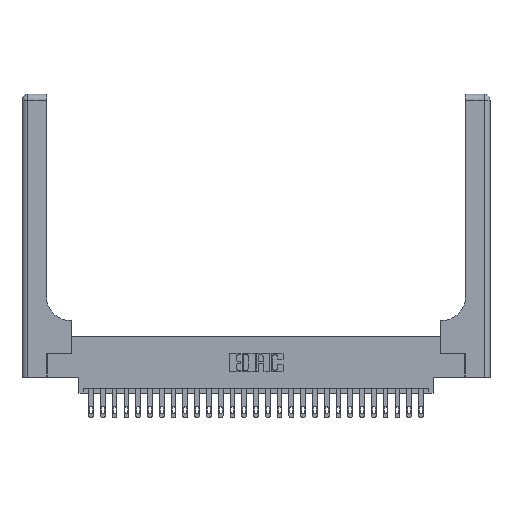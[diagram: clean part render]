
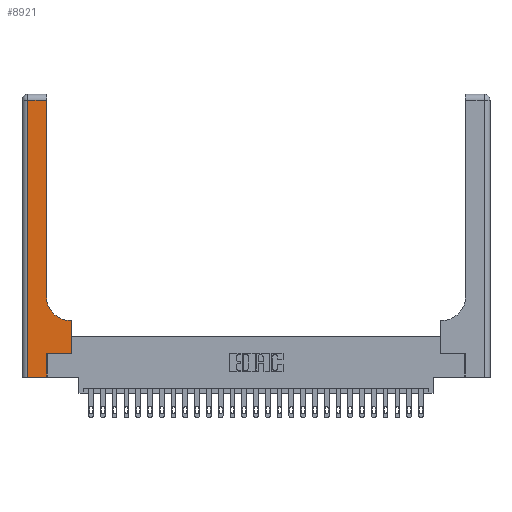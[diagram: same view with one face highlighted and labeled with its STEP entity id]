
A CAD part, top view. The second image highlights one B-rep face of the part: STEP entity #8921.
In plain terms, the highlighted planar face has unit normal (0, 0, 1).
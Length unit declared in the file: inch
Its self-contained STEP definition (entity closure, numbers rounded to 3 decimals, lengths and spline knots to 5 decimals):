
#951 = VECTOR ( 'NONE', #7399, 39.37008 ) ;
#977 = VERTEX_POINT ( 'NONE', #7825 ) ;
#1248 = EDGE_CURVE ( 'NONE', #22146, #21912, #2877, .T. ) ;
#1373 = VERTEX_POINT ( 'NONE', #18196 ) ;
#1767 = DIRECTION ( 'NONE',  ( -1., 0., 0. ) ) ;
#2043 = LINE ( 'NONE', #6017, #7101 ) ;
#2155 = EDGE_CURVE ( 'NONE', #2946, #977, #9315, .T. ) ;
#2622 = VERTEX_POINT ( 'NONE', #16186 ) ;
#2779 = AXIS2_PLACEMENT_3D ( 'NONE', #13784, #5751, #1767 ) ;
#2877 = LINE ( 'NONE', #7270, #951 ) ;
#2890 = VECTOR ( 'NONE', #3100, 39.37008 ) ;
#2946 = VERTEX_POINT ( 'NONE', #5224 ) ;
#3078 = CARTESIAN_POINT ( 'NONE',  ( 0.265, 0., 0.37 ) ) ;
#3100 = DIRECTION ( 'NONE',  ( 0., 1., 0. ) ) ;
#3441 = DIRECTION ( 'NONE',  ( 0., 1., 0. ) ) ;
#3541 = EDGE_CURVE ( 'NONE', #21912, #2622, #9478, .T. ) ;
#4646 = EDGE_CURVE ( 'NONE', #1373, #24744, #10700, .T. ) ;
#4874 = VECTOR ( 'NONE', #7732, 39.37008 ) ;
#5224 = CARTESIAN_POINT ( 'NONE',  ( 0.265, 0.25, 0.37 ) ) ;
#5430 = CARTESIAN_POINT ( 'NONE',  ( 0.26, 3., 0.37 ) ) ;
#5453 = CARTESIAN_POINT ( 'NONE',  ( 0.06, 3., 0.37 ) ) ;
#5552 = CARTESIAN_POINT ( 'NONE',  ( 0.265, 0.25, 0.37 ) ) ;
#5617 = PLANE ( 'NONE',  #2779 ) ;
#5751 = DIRECTION ( 'NONE',  ( 0., 0., -1. ) ) ;
#5753 = DIRECTION ( 'NONE',  ( -1., 0., 0. ) ) ;
#5936 = VECTOR ( 'NONE', #3441, 39.37008 ) ;
#6017 = CARTESIAN_POINT ( 'NONE',  ( 0., 0., 0.37 ) ) ;
#6042 = ORIENTED_EDGE ( 'NONE', *, *, #19328, .T. ) ;
#6421 = DIRECTION ( 'NONE',  ( 1., 0., 0. ) ) ;
#6619 = CARTESIAN_POINT ( 'NONE',  ( 0.26, 2.94, 0.37 ) ) ;
#7101 = VECTOR ( 'NONE', #6421, 39.37008 ) ;
#7240 = LINE ( 'NONE', #13647, #16101 ) ;
#7270 = CARTESIAN_POINT ( 'NONE',  ( 0., 2.94, 0.37 ) ) ;
#7368 = ORIENTED_EDGE ( 'NONE', *, *, #4646, .T. ) ;
#7399 = DIRECTION ( 'NONE',  ( -1., 0., 0. ) ) ;
#7627 = LINE ( 'NONE', #11647, #2890 ) ;
#7711 = LINE ( 'NONE', #5430, #5936 ) ;
#7732 = DIRECTION ( 'NONE',  ( 0., -1., 0. ) ) ;
#7825 = CARTESIAN_POINT ( 'NONE',  ( 0.528, 0.25, 0.37 ) ) ;
#8031 = CARTESIAN_POINT ( 'NONE',  ( 0.26, 0.85, 0.37 ) ) ;
#8921 = ADVANCED_FACE ( 'NONE', ( #23918 ), #5617, .F. ) ;
#9315 = LINE ( 'NONE', #5552, #20582 ) ;
#9478 = LINE ( 'NONE', #5453, #4874 ) ;
#10700 = LINE ( 'NONE', #18826, #16828 ) ;
#11647 = CARTESIAN_POINT ( 'NONE',  ( 0.265, 0., 0.37 ) ) ;
#12503 = AXIS2_PLACEMENT_3D ( 'NONE', #19893, #16030, #13903 ) ;
#12936 = CARTESIAN_POINT ( 'NONE',  ( 0.06, 2.94, 0.37 ) ) ;
#13388 = ORIENTED_EDGE ( 'NONE', *, *, #2155, .T. ) ;
#13463 = EDGE_LOOP ( 'NONE', ( #17006, #22555, #25211, #17265, #23075, #13388, #6042, #7368, #22482 ) ) ;
#13647 = CARTESIAN_POINT ( 'NONE',  ( 0.528, 0.25, 0.37 ) ) ;
#13784 = CARTESIAN_POINT ( 'NONE',  ( 0., 3., 0.37 ) ) ;
#13903 = DIRECTION ( 'NONE',  ( 1., 0., 0. ) ) ;
#15294 = VERTEX_POINT ( 'NONE', #3078 ) ;
#16030 = DIRECTION ( 'NONE',  ( 0., 0., -1. ) ) ;
#16101 = VECTOR ( 'NONE', #21770, 39.37008 ) ;
#16186 = CARTESIAN_POINT ( 'NONE',  ( 0.06, 0., 0.37 ) ) ;
#16828 = VECTOR ( 'NONE', #5753, 39.37008 ) ;
#17006 = ORIENTED_EDGE ( 'NONE', *, *, #21974, .T. ) ;
#17265 = ORIENTED_EDGE ( 'NONE', *, *, #24298, .T. ) ;
#17365 = CARTESIAN_POINT ( 'NONE',  ( 0.51, 0.6, 0.37 ) ) ;
#17457 = DIRECTION ( 'NONE',  ( 1., 0., 0. ) ) ;
#18014 = EDGE_CURVE ( 'NONE', #24744, #21343, #21865, .T. ) ;
#18196 = CARTESIAN_POINT ( 'NONE',  ( 0.528, 0.6, 0.37 ) ) ;
#18826 = CARTESIAN_POINT ( 'NONE',  ( 0.26, 0.6, 0.37 ) ) ;
#19326 = EDGE_CURVE ( 'NONE', #15294, #2946, #7627, .T. ) ;
#19328 = EDGE_CURVE ( 'NONE', #977, #1373, #7240, .T. ) ;
#19893 = CARTESIAN_POINT ( 'NONE',  ( 0.51, 0.85, 0.37 ) ) ;
#20582 = VECTOR ( 'NONE', #17457, 39.37008 ) ;
#21343 = VERTEX_POINT ( 'NONE', #8031 ) ;
#21770 = DIRECTION ( 'NONE',  ( 0., 1., 0. ) ) ;
#21865 = CIRCLE ( 'NONE', #12503, 0.25 ) ;
#21912 = VERTEX_POINT ( 'NONE', #12936 ) ;
#21974 = EDGE_CURVE ( 'NONE', #21343, #22146, #7711, .T. ) ;
#22146 = VERTEX_POINT ( 'NONE', #6619 ) ;
#22482 = ORIENTED_EDGE ( 'NONE', *, *, #18014, .T. ) ;
#22555 = ORIENTED_EDGE ( 'NONE', *, *, #1248, .T. ) ;
#23075 = ORIENTED_EDGE ( 'NONE', *, *, #19326, .T. ) ;
#23918 = FACE_OUTER_BOUND ( 'NONE', #13463, .T. ) ;
#24298 = EDGE_CURVE ( 'NONE', #2622, #15294, #2043, .T. ) ;
#24744 = VERTEX_POINT ( 'NONE', #17365 ) ;
#25211 = ORIENTED_EDGE ( 'NONE', *, *, #3541, .T. ) ;
